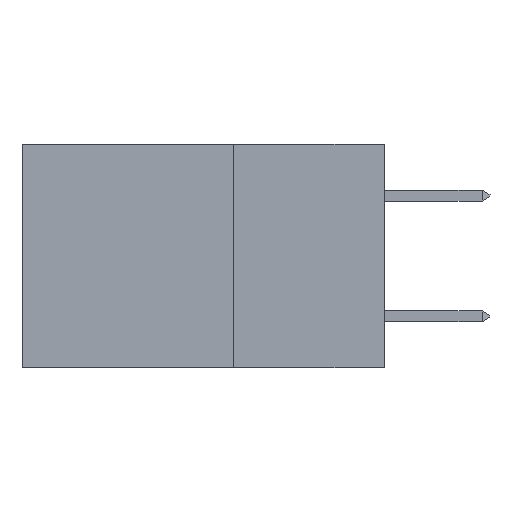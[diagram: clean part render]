
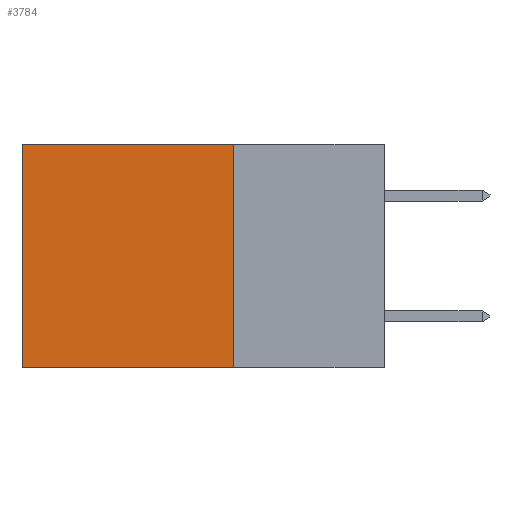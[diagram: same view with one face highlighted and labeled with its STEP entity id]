
A CAD part, left-side view. The second image highlights one B-rep face of the part: STEP entity #3784.
In plain terms, the highlighted planar face has unit normal (-1, 0, 0).
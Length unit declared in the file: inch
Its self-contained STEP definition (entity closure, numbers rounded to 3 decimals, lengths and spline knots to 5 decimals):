
#55 = VERTEX_POINT ( 'NONE', #6446 ) ;
#56 = ORIENTED_EDGE ( 'NONE', *, *, #5364, .F. ) ;
#185 = VERTEX_POINT ( 'NONE', #574 ) ;
#574 = CARTESIAN_POINT ( 'NONE',  ( 0.2875, 0.6, 0. ) ) ;
#1065 = VERTEX_POINT ( 'NONE', #8686 ) ;
#1102 = EDGE_LOOP ( 'NONE', ( #6825, #1939, #56, #2990 ) ) ;
#1939 = ORIENTED_EDGE ( 'NONE', *, *, #7250, .F. ) ;
#2275 = VECTOR ( 'NONE', #11129, 39.37008 ) ;
#2409 = DIRECTION ( 'NONE',  ( 0., 1., 0. ) ) ;
#2564 = AXIS2_PLACEMENT_3D ( 'NONE', #8239, #9123, #3843 ) ;
#2947 = CARTESIAN_POINT ( 'NONE',  ( 0.2875, 0.25, 0. ) ) ;
#2990 = ORIENTED_EDGE ( 'NONE', *, *, #10036, .T. ) ;
#3263 = LINE ( 'NONE', #10180, #2275 ) ;
#3547 = LINE ( 'NONE', #2947, #6007 ) ;
#3784 = ADVANCED_FACE ( 'NONE', ( #8111 ), #7352, .F. ) ;
#3843 = DIRECTION ( 'NONE',  ( 0., 0., -1. ) ) ;
#3975 = CARTESIAN_POINT ( 'NONE',  ( 0.2875, 0.6, 0. ) ) ;
#5364 = EDGE_CURVE ( 'NONE', #55, #8779, #3547, .T. ) ;
#5407 = VECTOR ( 'NONE', #2409, 39.37008 ) ;
#5582 = LINE ( 'NONE', #3975, #5999 ) ;
#5999 = VECTOR ( 'NONE', #11178, 39.37008 ) ;
#6007 = VECTOR ( 'NONE', #8238, 39.37008 ) ;
#6446 = CARTESIAN_POINT ( 'NONE',  ( 0.2875, 0.25, 0. ) ) ;
#6825 = ORIENTED_EDGE ( 'NONE', *, *, #9382, .T. ) ;
#7250 = EDGE_CURVE ( 'NONE', #8779, #1065, #9598, .T. ) ;
#7352 = PLANE ( 'NONE',  #2564 ) ;
#7665 = CARTESIAN_POINT ( 'NONE',  ( 0.2875, 0.25, -0.37 ) ) ;
#8111 = FACE_OUTER_BOUND ( 'NONE', #1102, .T. ) ;
#8238 = DIRECTION ( 'NONE',  ( 0., 0., -1. ) ) ;
#8239 = CARTESIAN_POINT ( 'NONE',  ( 0.2875, 0.25, 0. ) ) ;
#8686 = CARTESIAN_POINT ( 'NONE',  ( 0.2875, 0.6, -0.37 ) ) ;
#8779 = VERTEX_POINT ( 'NONE', #9490 ) ;
#9123 = DIRECTION ( 'NONE',  ( 1., 0., 0. ) ) ;
#9382 = EDGE_CURVE ( 'NONE', #185, #1065, #5582, .T. ) ;
#9490 = CARTESIAN_POINT ( 'NONE',  ( 0.2875, 0.25, -0.37 ) ) ;
#9598 = LINE ( 'NONE', #7665, #5407 ) ;
#10036 = EDGE_CURVE ( 'NONE', #55, #185, #3263, .T. ) ;
#10180 = CARTESIAN_POINT ( 'NONE',  ( 0.2875, 0.25, 0. ) ) ;
#11129 = DIRECTION ( 'NONE',  ( 0., 1., 0. ) ) ;
#11178 = DIRECTION ( 'NONE',  ( 0., 0., -1. ) ) ;
